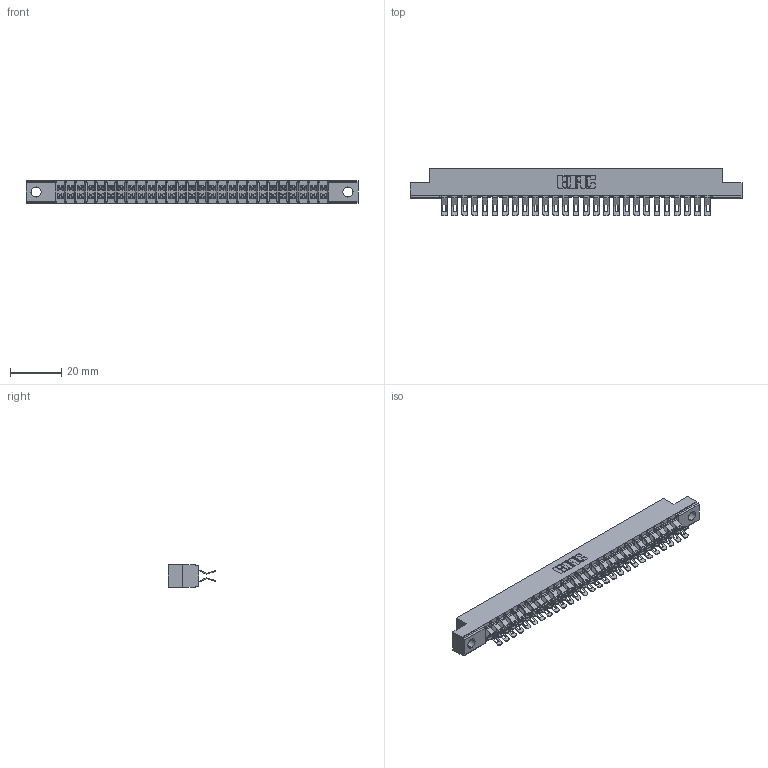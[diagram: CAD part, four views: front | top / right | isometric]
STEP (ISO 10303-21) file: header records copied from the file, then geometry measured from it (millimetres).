
FILE_DESCRIPTION (( 'STEP AP203' ), '1' );
FILE_NAME ('357-054-455-204.STEP', '2020-10-04T08:55:02', ( '' ), ( '' ), 'SwSTEP 2.0', 'SolidWorks 2020', '' );
FILE_SCHEMA (( 'CONFIG_CONTROL_DESIGN' ));
Length unit declared in the file: inch
Products named in the file (3): 357-054-455-204; 307-290-001_555; 307 Part_.156 Dia Mounting Holes
Assembly tree (55 placements, depth 2):
  357-054-455-204
    307 Part_.156 Dia Mounting Holes
    307-290-001_555  x54
Bounding box: 130 x 18.75 x 8.71 mm (x, y, z)
Volume: 8557.6 mm3; surface area: 16152.6 mm2
Topology: 55 solids, 55 shells, 3454 faces, 10133 edges, 6606 vertices
Faces by surface type: plane 1920, cylinder 1478, sphere 56
Entity records: 26815 total; most frequent: CARTESIAN_POINT 4401, ORIENTED_EDGE 4360, DIRECTION 4316, EDGE_CURVE 2180, LINE 1662, VECTOR 1662, VERTEX_POINT 1412, AXIS2_PLACEMENT_3D 1327
